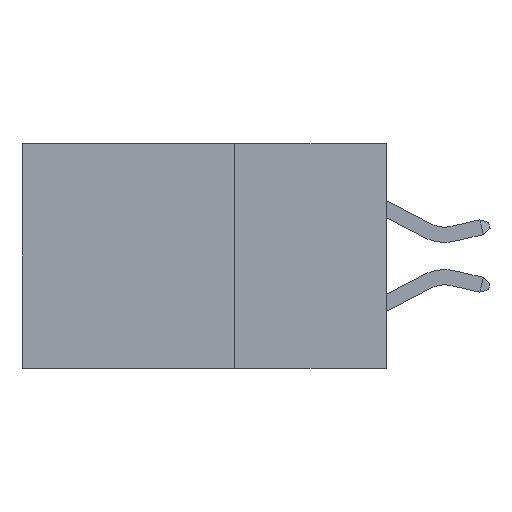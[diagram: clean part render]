
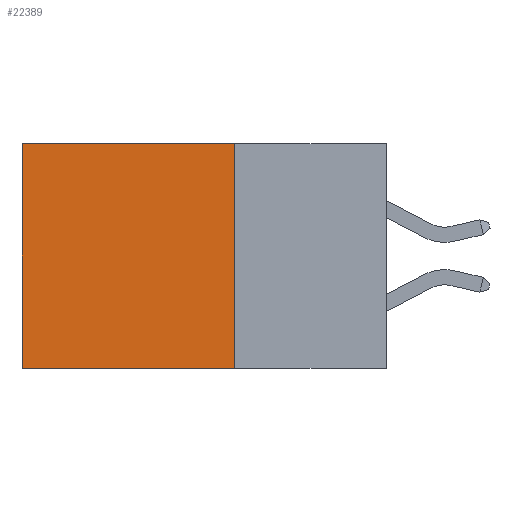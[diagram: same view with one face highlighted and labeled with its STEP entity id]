
A CAD part, left-side view. The second image highlights one B-rep face of the part: STEP entity #22389.
In plain terms, the highlighted planar face has unit normal (-1, 0, 0).
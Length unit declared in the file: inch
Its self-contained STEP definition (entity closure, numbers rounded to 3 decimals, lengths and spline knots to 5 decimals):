
#198 = VECTOR ( 'NONE', #6529, 39.37008 ) ;
#1027 = ORIENTED_EDGE ( 'NONE', *, *, #7233, .T. ) ;
#1726 = LINE ( 'NONE', #5595, #10721 ) ;
#1976 = VERTEX_POINT ( 'NONE', #15381 ) ;
#2536 = DIRECTION ( 'NONE',  ( 1., 0., 0. ) ) ;
#2627 = EDGE_CURVE ( 'NONE', #9195, #16474, #21326, .T. ) ;
#2767 = CARTESIAN_POINT ( 'NONE',  ( 0.298, 0.6, 0. ) ) ;
#4635 = AXIS2_PLACEMENT_3D ( 'NONE', #7887, #2536, #15035 ) ;
#5595 = CARTESIAN_POINT ( 'NONE',  ( 0.298, 0.25, -0.37 ) ) ;
#6529 = DIRECTION ( 'NONE',  ( 0., 1., 0. ) ) ;
#7161 = EDGE_LOOP ( 'NONE', ( #19033, #15539, #15510, #1027 ) ) ;
#7233 = EDGE_CURVE ( 'NONE', #22004, #9195, #9810, .T. ) ;
#7887 = CARTESIAN_POINT ( 'NONE',  ( 0.298, 0.25, 0. ) ) ;
#9195 = VERTEX_POINT ( 'NONE', #2767 ) ;
#9810 = LINE ( 'NONE', #18896, #198 ) ;
#10721 = VECTOR ( 'NONE', #17979, 39.37008 ) ;
#11099 = EDGE_CURVE ( 'NONE', #22004, #1976, #11402, .T. ) ;
#11402 = LINE ( 'NONE', #20941, #15511 ) ;
#12269 = FACE_OUTER_BOUND ( 'NONE', #7161, .T. ) ;
#13268 = PLANE ( 'NONE',  #4635 ) ;
#13282 = EDGE_CURVE ( 'NONE', #1976, #16474, #1726, .T. ) ;
#14695 = CARTESIAN_POINT ( 'NONE',  ( 0.298, 0.6, 0. ) ) ;
#15035 = DIRECTION ( 'NONE',  ( 0., 0., -1. ) ) ;
#15381 = CARTESIAN_POINT ( 'NONE',  ( 0.298, 0.25, -0.37 ) ) ;
#15510 = ORIENTED_EDGE ( 'NONE', *, *, #11099, .F. ) ;
#15511 = VECTOR ( 'NONE', #22739, 39.37008 ) ;
#15539 = ORIENTED_EDGE ( 'NONE', *, *, #13282, .F. ) ;
#16474 = VERTEX_POINT ( 'NONE', #19703 ) ;
#17979 = DIRECTION ( 'NONE',  ( 0., 1., 0. ) ) ;
#18896 = CARTESIAN_POINT ( 'NONE',  ( 0.298, 0.25, 0. ) ) ;
#19033 = ORIENTED_EDGE ( 'NONE', *, *, #2627, .T. ) ;
#19401 = VECTOR ( 'NONE', #19683, 39.37008 ) ;
#19683 = DIRECTION ( 'NONE',  ( 0., 0., -1. ) ) ;
#19703 = CARTESIAN_POINT ( 'NONE',  ( 0.298, 0.6, -0.37 ) ) ;
#20941 = CARTESIAN_POINT ( 'NONE',  ( 0.298, 0.25, 0. ) ) ;
#21107 = CARTESIAN_POINT ( 'NONE',  ( 0.298, 0.25, 0. ) ) ;
#21326 = LINE ( 'NONE', #14695, #19401 ) ;
#22004 = VERTEX_POINT ( 'NONE', #21107 ) ;
#22389 = ADVANCED_FACE ( 'NONE', ( #12269 ), #13268, .F. ) ;
#22739 = DIRECTION ( 'NONE',  ( 0., 0., -1. ) ) ;
